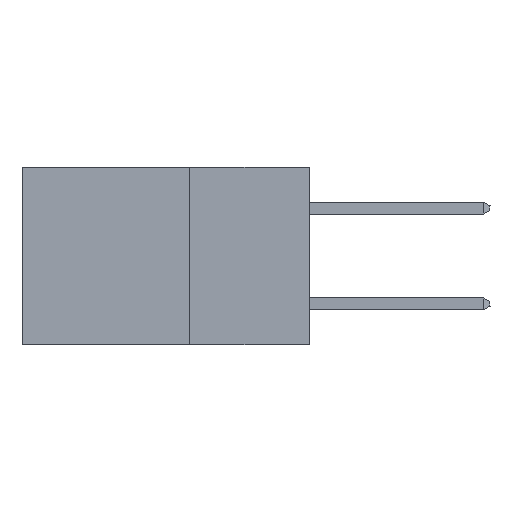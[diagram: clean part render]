
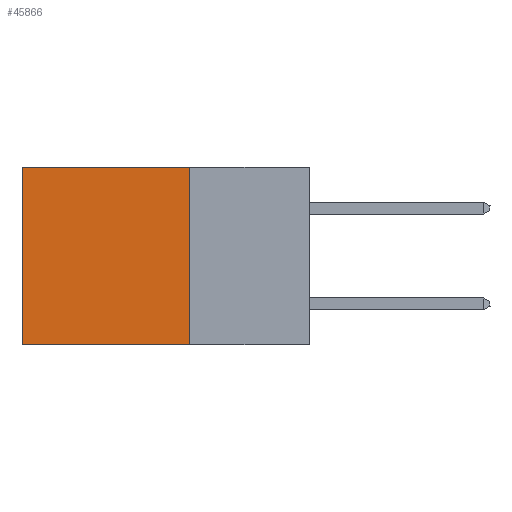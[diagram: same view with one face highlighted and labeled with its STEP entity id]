
A CAD part, left-side view. The second image highlights one B-rep face of the part: STEP entity #45866.
In plain terms, the highlighted planar face has unit normal (-1, 0, 0).
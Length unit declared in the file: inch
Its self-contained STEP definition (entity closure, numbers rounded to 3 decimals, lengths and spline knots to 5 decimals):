
#2003 = ORIENTED_EDGE ( 'NONE', *, *, #32974, .T. ) ;
#2665 = CARTESIAN_POINT ( 'NONE',  ( 0.2875, 0.25, 0. ) ) ;
#3457 = CARTESIAN_POINT ( 'NONE',  ( 0.2875, 0.25, 0. ) ) ;
#4566 = VECTOR ( 'NONE', #14725, 39.37008 ) ;
#6278 = DIRECTION ( 'NONE',  ( 1., 0., 0. ) ) ;
#6298 = VECTOR ( 'NONE', #43091, 39.37008 ) ;
#9127 = EDGE_CURVE ( 'NONE', #12114, #45405, #24317, .T. ) ;
#9383 = VECTOR ( 'NONE', #9986, 39.37008 ) ;
#9986 = DIRECTION ( 'NONE',  ( 0., 1., 0. ) ) ;
#11013 = EDGE_LOOP ( 'NONE', ( #2003, #14868, #16792, #35629 ) ) ;
#12114 = VERTEX_POINT ( 'NONE', #3457 ) ;
#14544 = CARTESIAN_POINT ( 'NONE',  ( 0.2875, 0.25, -0.37 ) ) ;
#14725 = DIRECTION ( 'NONE',  ( 0., 0., -1. ) ) ;
#14779 = VERTEX_POINT ( 'NONE', #14913 ) ;
#14868 = ORIENTED_EDGE ( 'NONE', *, *, #22299, .F. ) ;
#14913 = CARTESIAN_POINT ( 'NONE',  ( 0.2875, 0.6, 0. ) ) ;
#15982 = DIRECTION ( 'NONE',  ( 0., 1., 0. ) ) ;
#16102 = FACE_OUTER_BOUND ( 'NONE', #11013, .T. ) ;
#16792 = ORIENTED_EDGE ( 'NONE', *, *, #9127, .F. ) ;
#17474 = VECTOR ( 'NONE', #15982, 39.37008 ) ;
#19855 = VERTEX_POINT ( 'NONE', #31225 ) ;
#20902 = LINE ( 'NONE', #21808, #4566 ) ;
#21808 = CARTESIAN_POINT ( 'NONE',  ( 0.2875, 0.6, 0. ) ) ;
#22299 = EDGE_CURVE ( 'NONE', #45405, #19855, #36467, .T. ) ;
#22539 = LINE ( 'NONE', #37607, #17474 ) ;
#24317 = LINE ( 'NONE', #24812, #6298 ) ;
#24812 = CARTESIAN_POINT ( 'NONE',  ( 0.2875, 0.25, 0. ) ) ;
#29410 = AXIS2_PLACEMENT_3D ( 'NONE', #2665, #6278, #31499 ) ;
#31225 = CARTESIAN_POINT ( 'NONE',  ( 0.2875, 0.6, -0.37 ) ) ;
#31499 = DIRECTION ( 'NONE',  ( 0., 0., -1. ) ) ;
#32974 = EDGE_CURVE ( 'NONE', #14779, #19855, #20902, .T. ) ;
#35629 = ORIENTED_EDGE ( 'NONE', *, *, #43555, .T. ) ;
#36467 = LINE ( 'NONE', #41193, #9383 ) ;
#37607 = CARTESIAN_POINT ( 'NONE',  ( 0.2875, 0.25, 0. ) ) ;
#41193 = CARTESIAN_POINT ( 'NONE',  ( 0.2875, 0.25, -0.37 ) ) ;
#42190 = PLANE ( 'NONE',  #29410 ) ;
#43091 = DIRECTION ( 'NONE',  ( 0., 0., -1. ) ) ;
#43555 = EDGE_CURVE ( 'NONE', #12114, #14779, #22539, .T. ) ;
#45405 = VERTEX_POINT ( 'NONE', #14544 ) ;
#45866 = ADVANCED_FACE ( 'NONE', ( #16102 ), #42190, .F. ) ;
